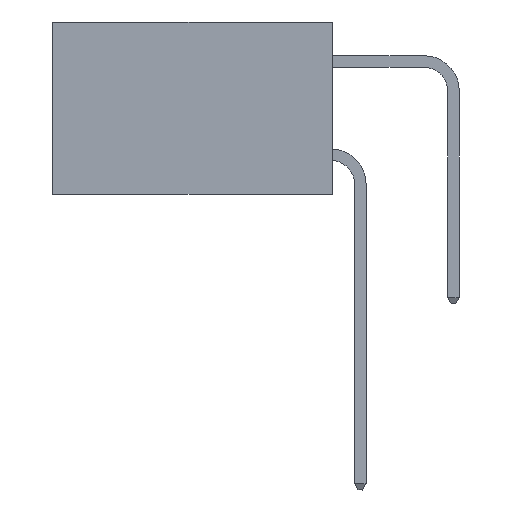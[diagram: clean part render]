
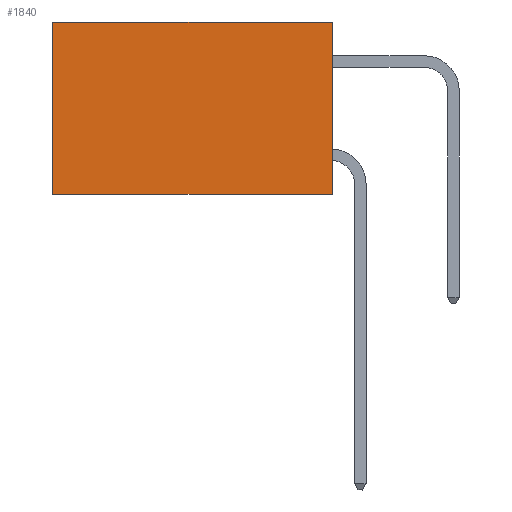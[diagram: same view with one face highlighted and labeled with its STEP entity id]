
A CAD part, left-side view. The second image highlights one B-rep face of the part: STEP entity #1840.
In plain terms, the highlighted planar face has unit normal (-1, 0, 0).
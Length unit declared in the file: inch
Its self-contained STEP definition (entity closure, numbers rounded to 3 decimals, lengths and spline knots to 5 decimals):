
#104 = EDGE_CURVE ( 'NONE', #6271, #17114, #5722, .T. ) ;
#271 = CARTESIAN_POINT ( 'NONE',  ( 0.2615, 0., -0.37 ) ) ;
#921 = VECTOR ( 'NONE', #14917, 39.37008 ) ;
#1538 = VECTOR ( 'NONE', #3464, 39.37008 ) ;
#1618 = FACE_OUTER_BOUND ( 'NONE', #13235, .T. ) ;
#1696 = LINE ( 'NONE', #14002, #1538 ) ;
#1815 = PLANE ( 'NONE',  #11353 ) ;
#1840 = ADVANCED_FACE ( 'NONE', ( #1618 ), #1815, .F. ) ;
#3058 = DIRECTION ( 'NONE',  ( 0., 0., -1. ) ) ;
#3464 = DIRECTION ( 'NONE',  ( 0., 0., -1. ) ) ;
#5518 = CARTESIAN_POINT ( 'NONE',  ( 0.2615, 0.6, -0.37 ) ) ;
#5722 = LINE ( 'NONE', #11584, #19274 ) ;
#5798 = VECTOR ( 'NONE', #3058, 39.37008 ) ;
#5829 = CARTESIAN_POINT ( 'NONE',  ( 0.2615, 0., -0.37 ) ) ;
#6271 = VERTEX_POINT ( 'NONE', #6967 ) ;
#6411 = ORIENTED_EDGE ( 'NONE', *, *, #7485, .T. ) ;
#6967 = CARTESIAN_POINT ( 'NONE',  ( 0.2615, 0., 0. ) ) ;
#7485 = EDGE_CURVE ( 'NONE', #17114, #7997, #1696, .T. ) ;
#7997 = VERTEX_POINT ( 'NONE', #5518 ) ;
#9118 = LINE ( 'NONE', #16545, #5798 ) ;
#9788 = EDGE_CURVE ( 'NONE', #14348, #7997, #10270, .T. ) ;
#10003 = CARTESIAN_POINT ( 'NONE',  ( 0.2615, 0.6, 0. ) ) ;
#10270 = LINE ( 'NONE', #13648, #921 ) ;
#10340 = DIRECTION ( 'NONE',  ( 1., 0., 0. ) ) ;
#10613 = DIRECTION ( 'NONE',  ( 0., 0., -1. ) ) ;
#11353 = AXIS2_PLACEMENT_3D ( 'NONE', #5829, #10340, #10613 ) ;
#11483 = EDGE_CURVE ( 'NONE', #6271, #14348, #9118, .T. ) ;
#11584 = CARTESIAN_POINT ( 'NONE',  ( 0.2615, 0., 0. ) ) ;
#13206 = DIRECTION ( 'NONE',  ( 0., 1., 0. ) ) ;
#13235 = EDGE_LOOP ( 'NONE', ( #6411, #14171, #16112, #17046 ) ) ;
#13648 = CARTESIAN_POINT ( 'NONE',  ( 0.2615, 0., -0.37 ) ) ;
#14002 = CARTESIAN_POINT ( 'NONE',  ( 0.2615, 0.6, -0.37 ) ) ;
#14171 = ORIENTED_EDGE ( 'NONE', *, *, #9788, .F. ) ;
#14348 = VERTEX_POINT ( 'NONE', #271 ) ;
#14917 = DIRECTION ( 'NONE',  ( 0., 1., 0. ) ) ;
#16112 = ORIENTED_EDGE ( 'NONE', *, *, #11483, .F. ) ;
#16545 = CARTESIAN_POINT ( 'NONE',  ( 0.2615, 0., -0.37 ) ) ;
#17046 = ORIENTED_EDGE ( 'NONE', *, *, #104, .T. ) ;
#17114 = VERTEX_POINT ( 'NONE', #10003 ) ;
#19274 = VECTOR ( 'NONE', #13206, 39.37008 ) ;
